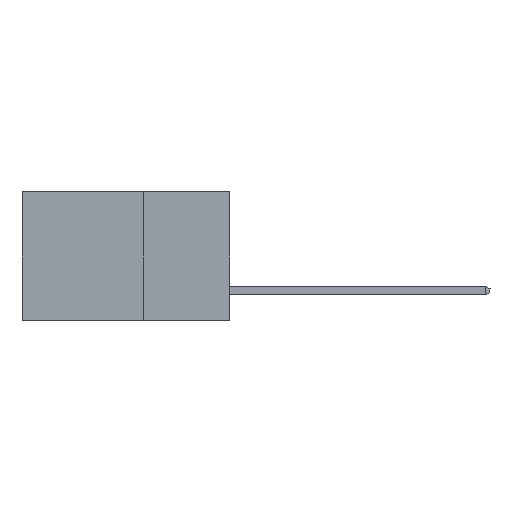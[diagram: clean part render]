
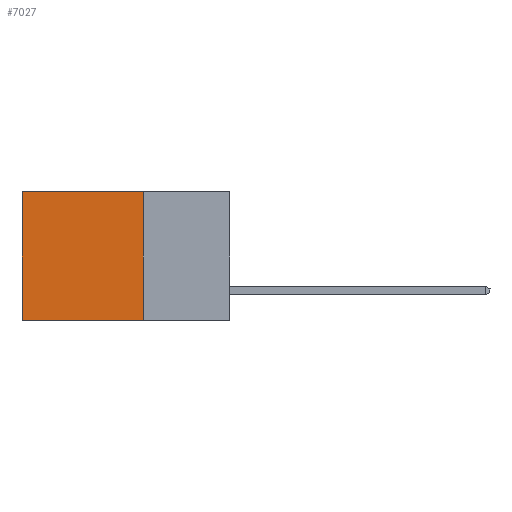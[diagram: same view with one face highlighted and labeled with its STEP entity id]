
A CAD part, left-side view. The second image highlights one B-rep face of the part: STEP entity #7027.
In plain terms, the highlighted planar face has unit normal (-1, 0, 0).
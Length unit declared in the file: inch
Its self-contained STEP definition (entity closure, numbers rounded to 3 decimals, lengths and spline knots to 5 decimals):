
#821 = DIRECTION ( 'NONE',  ( 0., 0., -1. ) ) ;
#846 = CARTESIAN_POINT ( 'NONE',  ( 0.2615, 0.6, 0. ) ) ;
#1160 = PLANE ( 'NONE',  #9417 ) ;
#2627 = VERTEX_POINT ( 'NONE', #846 ) ;
#2635 = VECTOR ( 'NONE', #13066, 39.37008 ) ;
#3139 = EDGE_CURVE ( 'NONE', #9266, #2627, #5766, .T. ) ;
#3855 = FACE_OUTER_BOUND ( 'NONE', #6160, .T. ) ;
#4334 = LINE ( 'NONE', #8406, #13008 ) ;
#4573 = DIRECTION ( 'NONE',  ( 0., 0., -1. ) ) ;
#4956 = EDGE_CURVE ( 'NONE', #6262, #12879, #4334, .T. ) ;
#5527 = EDGE_CURVE ( 'NONE', #9266, #6262, #9772, .T. ) ;
#5766 = LINE ( 'NONE', #10880, #2635 ) ;
#6160 = EDGE_LOOP ( 'NONE', ( #10022, #7976, #11318, #10024 ) ) ;
#6262 = VERTEX_POINT ( 'NONE', #8481 ) ;
#7027 = ADVANCED_FACE ( 'NONE', ( #3855 ), #1160, .F. ) ;
#7249 = CARTESIAN_POINT ( 'NONE',  ( 0.2615, 0.6, -0.37 ) ) ;
#7436 = DIRECTION ( 'NONE',  ( 0., 1., 0. ) ) ;
#7976 = ORIENTED_EDGE ( 'NONE', *, *, #4956, .F. ) ;
#8406 = CARTESIAN_POINT ( 'NONE',  ( 0.2615, 0.25, -0.37 ) ) ;
#8481 = CARTESIAN_POINT ( 'NONE',  ( 0.2615, 0.25, -0.37 ) ) ;
#8894 = EDGE_CURVE ( 'NONE', #2627, #12879, #10442, .T. ) ;
#9266 = VERTEX_POINT ( 'NONE', #9338 ) ;
#9338 = CARTESIAN_POINT ( 'NONE',  ( 0.2615, 0.25, 0. ) ) ;
#9417 = AXIS2_PLACEMENT_3D ( 'NONE', #10454, #12429, #10788 ) ;
#9772 = LINE ( 'NONE', #10961, #10055 ) ;
#10022 = ORIENTED_EDGE ( 'NONE', *, *, #8894, .T. ) ;
#10024 = ORIENTED_EDGE ( 'NONE', *, *, #3139, .T. ) ;
#10055 = VECTOR ( 'NONE', #4573, 39.37008 ) ;
#10442 = LINE ( 'NONE', #12560, #13053 ) ;
#10454 = CARTESIAN_POINT ( 'NONE',  ( 0.2615, 0.25, -0.37 ) ) ;
#10788 = DIRECTION ( 'NONE',  ( 0., 0., -1. ) ) ;
#10880 = CARTESIAN_POINT ( 'NONE',  ( 0.2615, 0.25, 0. ) ) ;
#10961 = CARTESIAN_POINT ( 'NONE',  ( 0.2615, 0.25, -0.37 ) ) ;
#11318 = ORIENTED_EDGE ( 'NONE', *, *, #5527, .F. ) ;
#12429 = DIRECTION ( 'NONE',  ( 1., 0., 0. ) ) ;
#12560 = CARTESIAN_POINT ( 'NONE',  ( 0.2615, 0.6, -0.37 ) ) ;
#12879 = VERTEX_POINT ( 'NONE', #7249 ) ;
#13008 = VECTOR ( 'NONE', #7436, 39.37008 ) ;
#13053 = VECTOR ( 'NONE', #821, 39.37008 ) ;
#13066 = DIRECTION ( 'NONE',  ( 0., 1., 0. ) ) ;
